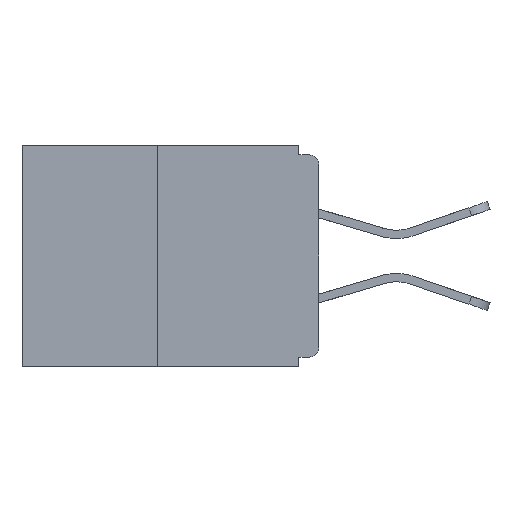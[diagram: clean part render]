
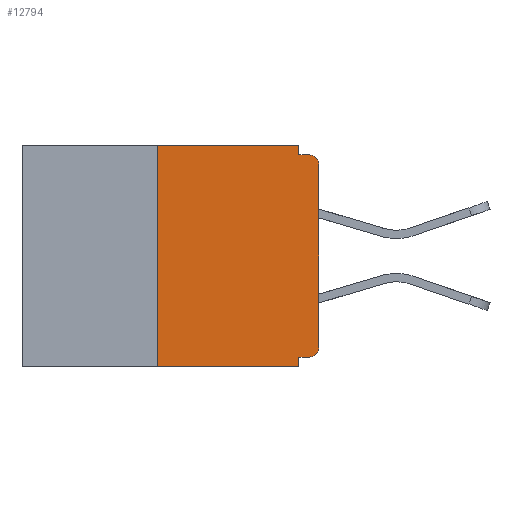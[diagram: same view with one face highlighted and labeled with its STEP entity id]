
A CAD part, left-side view. The second image highlights one B-rep face of the part: STEP entity #12794.
In plain terms, the highlighted planar face has unit normal (-1, 0, 0).
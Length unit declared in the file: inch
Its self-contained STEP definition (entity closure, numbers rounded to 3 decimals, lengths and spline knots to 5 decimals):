
#312 = VERTEX_POINT ( 'NONE', #1447 ) ;
#1018 = DIRECTION ( 'NONE',  ( 0., 0., 1. ) ) ;
#1177 = LINE ( 'NONE', #8014, #24365 ) ;
#1422 = LINE ( 'NONE', #25446, #17984 ) ;
#1447 = CARTESIAN_POINT ( 'NONE',  ( 0., 0.015, -0.328 ) ) ;
#1705 = CARTESIAN_POINT ( 'NONE',  ( 0., 0.031, 0. ) ) ;
#1796 = PLANE ( 'NONE',  #27932 ) ;
#2802 = AXIS2_PLACEMENT_3D ( 'NONE', #18788, #21518, #6043 ) ;
#3349 = ORIENTED_EDGE ( 'NONE', *, *, #22629, .F. ) ;
#3696 = VECTOR ( 'NONE', #6148, 39.37008 ) ;
#3908 = VERTEX_POINT ( 'NONE', #17465 ) ;
#4246 = CARTESIAN_POINT ( 'NONE',  ( 0., 0.25, -0.343 ) ) ;
#4397 = ORIENTED_EDGE ( 'NONE', *, *, #15735, .T. ) ;
#4844 = VERTEX_POINT ( 'NONE', #19681 ) ;
#5468 = EDGE_CURVE ( 'NONE', #14798, #24019, #1177, .T. ) ;
#6002 = DIRECTION ( 'NONE',  ( -1., 0., 0. ) ) ;
#6043 = DIRECTION ( 'NONE',  ( 0., 0., -1. ) ) ;
#6148 = DIRECTION ( 'NONE',  ( 0., -1., 0. ) ) ;
#6661 = VERTEX_POINT ( 'NONE', #7827 ) ;
#6796 = VERTEX_POINT ( 'NONE', #1705 ) ;
#7827 = CARTESIAN_POINT ( 'NONE',  ( 0., 0.015, -0.015 ) ) ;
#8014 = CARTESIAN_POINT ( 'NONE',  ( 0., 0., 0. ) ) ;
#8288 = DIRECTION ( 'NONE',  ( 0., 0., -1. ) ) ;
#8765 = CARTESIAN_POINT ( 'NONE',  ( 0., 0., -0.328 ) ) ;
#8802 = EDGE_LOOP ( 'NONE', ( #13668, #12672, #10462, #15686, #23230, #9594, #11834, #4397, #16096, #3349 ) ) ;
#9047 = DIRECTION ( 'NONE',  ( 0., -1., 0. ) ) ;
#9594 = ORIENTED_EDGE ( 'NONE', *, *, #16362, .T. ) ;
#9711 = EDGE_CURVE ( 'NONE', #3908, #6796, #14964, .T. ) ;
#10166 = LINE ( 'NONE', #22773, #10585 ) ;
#10358 = DIRECTION ( 'NONE',  ( 1., 0., 0. ) ) ;
#10462 = ORIENTED_EDGE ( 'NONE', *, *, #19472, .T. ) ;
#10585 = VECTOR ( 'NONE', #14324, 39.37008 ) ;
#10983 = AXIS2_PLACEMENT_3D ( 'NONE', #23483, #6002, #8288 ) ;
#11169 = CARTESIAN_POINT ( 'NONE',  ( 0., 0.031, -0.015 ) ) ;
#11596 = DIRECTION ( 'NONE',  ( 0., 0., -1. ) ) ;
#11744 = LINE ( 'NONE', #26909, #25302 ) ;
#11834 = ORIENTED_EDGE ( 'NONE', *, *, #5468, .T. ) ;
#11991 = DIRECTION ( 'NONE',  ( 0., 0., -1. ) ) ;
#12185 = VERTEX_POINT ( 'NONE', #17697 ) ;
#12245 = CARTESIAN_POINT ( 'NONE',  ( 0., 0., -0.313 ) ) ;
#12672 = ORIENTED_EDGE ( 'NONE', *, *, #20843, .F. ) ;
#12794 = ADVANCED_FACE ( 'NONE', ( #21906 ), #1796, .F. ) ;
#13654 = DIRECTION ( 'NONE',  ( 0., 1., 0. ) ) ;
#13668 = ORIENTED_EDGE ( 'NONE', *, *, #9711, .F. ) ;
#13782 = VERTEX_POINT ( 'NONE', #4246 ) ;
#14324 = DIRECTION ( 'NONE',  ( 0., 0., 1. ) ) ;
#14798 = VERTEX_POINT ( 'NONE', #12245 ) ;
#14820 = DIRECTION ( 'NONE',  ( 0., -1., 0. ) ) ;
#14964 = LINE ( 'NONE', #23701, #24011 ) ;
#15503 = CARTESIAN_POINT ( 'NONE',  ( 0., 0.46, -0.343 ) ) ;
#15677 = EDGE_CURVE ( 'NONE', #20526, #6661, #16183, .T. ) ;
#15686 = ORIENTED_EDGE ( 'NONE', *, *, #18844, .F. ) ;
#15735 = EDGE_CURVE ( 'NONE', #24019, #6661, #19671, .T. ) ;
#16096 = ORIENTED_EDGE ( 'NONE', *, *, #15677, .F. ) ;
#16183 = LINE ( 'NONE', #22770, #3696 ) ;
#16362 = EDGE_CURVE ( 'NONE', #312, #14798, #16980, .T. ) ;
#16980 = CIRCLE ( 'NONE', #2802, 0.015 ) ;
#17099 = DIRECTION ( 'NONE',  ( 0., 0., -1. ) ) ;
#17416 = EDGE_CURVE ( 'NONE', #312, #12185, #19661, .T. ) ;
#17465 = CARTESIAN_POINT ( 'NONE',  ( 0., 0.25, 0. ) ) ;
#17697 = CARTESIAN_POINT ( 'NONE',  ( 0., 0.031, -0.328 ) ) ;
#17733 = CARTESIAN_POINT ( 'NONE',  ( 0., 0., -0.03 ) ) ;
#17984 = VECTOR ( 'NONE', #11991, 39.37008 ) ;
#18788 = CARTESIAN_POINT ( 'NONE',  ( 0., 0.015, -0.313 ) ) ;
#18844 = EDGE_CURVE ( 'NONE', #12185, #4844, #11744, .T. ) ;
#19472 = EDGE_CURVE ( 'NONE', #13782, #4844, #22246, .T. ) ;
#19661 = LINE ( 'NONE', #8765, #27069 ) ;
#19671 = CIRCLE ( 'NONE', #10983, 0.015 ) ;
#19681 = CARTESIAN_POINT ( 'NONE',  ( 0., 0.031, -0.343 ) ) ;
#20526 = VERTEX_POINT ( 'NONE', #11169 ) ;
#20843 = EDGE_CURVE ( 'NONE', #13782, #3908, #10166, .T. ) ;
#20963 = CARTESIAN_POINT ( 'NONE',  ( 0., 0.46, 0. ) ) ;
#21518 = DIRECTION ( 'NONE',  ( -1., 0., 0. ) ) ;
#21906 = FACE_OUTER_BOUND ( 'NONE', #8802, .T. ) ;
#22246 = LINE ( 'NONE', #15503, #27829 ) ;
#22629 = EDGE_CURVE ( 'NONE', #6796, #20526, #1422, .T. ) ;
#22770 = CARTESIAN_POINT ( 'NONE',  ( 0., 0., -0.015 ) ) ;
#22773 = CARTESIAN_POINT ( 'NONE',  ( 0., 0.25, 0. ) ) ;
#23230 = ORIENTED_EDGE ( 'NONE', *, *, #17416, .F. ) ;
#23483 = CARTESIAN_POINT ( 'NONE',  ( 0., 0.015, -0.03 ) ) ;
#23701 = CARTESIAN_POINT ( 'NONE',  ( 0., 0.46, 0. ) ) ;
#24011 = VECTOR ( 'NONE', #14820, 39.37008 ) ;
#24019 = VERTEX_POINT ( 'NONE', #17733 ) ;
#24365 = VECTOR ( 'NONE', #1018, 39.37008 ) ;
#25302 = VECTOR ( 'NONE', #11596, 39.37008 ) ;
#25446 = CARTESIAN_POINT ( 'NONE',  ( 0., 0.031, 0. ) ) ;
#26909 = CARTESIAN_POINT ( 'NONE',  ( 0., 0.031, -0.343 ) ) ;
#27069 = VECTOR ( 'NONE', #13654, 39.37008 ) ;
#27829 = VECTOR ( 'NONE', #9047, 39.37008 ) ;
#27932 = AXIS2_PLACEMENT_3D ( 'NONE', #20963, #10358, #17099 ) ;
